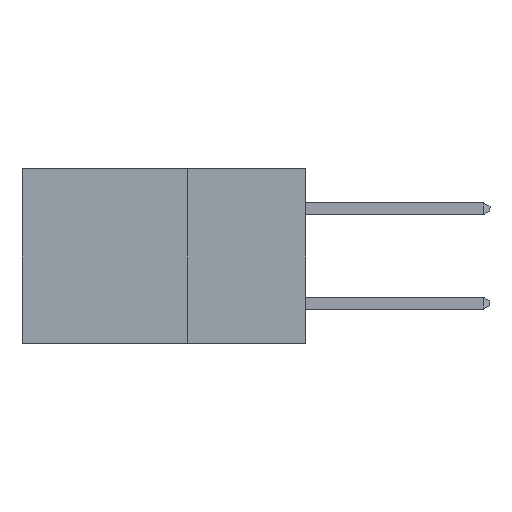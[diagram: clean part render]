
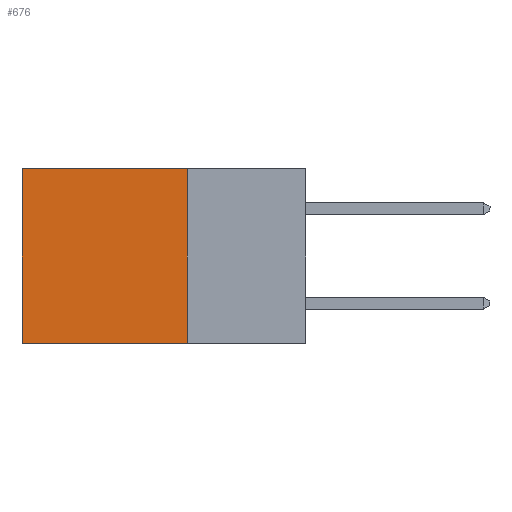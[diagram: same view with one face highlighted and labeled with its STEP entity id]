
A CAD part, left-side view. The second image highlights one B-rep face of the part: STEP entity #676.
In plain terms, the highlighted planar face has unit normal (-1, 0, 0).
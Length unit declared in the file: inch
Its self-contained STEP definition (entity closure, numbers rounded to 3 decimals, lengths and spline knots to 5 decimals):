
#16 = ORIENTED_EDGE ( 'NONE', *, *, #1226, .T. ) ;
#355 = CARTESIAN_POINT ( 'NONE',  ( 0.2615, 0.25, -0.37 ) ) ;
#676 = ADVANCED_FACE ( 'NONE', ( #8545 ), #761, .F. ) ;
#695 = VERTEX_POINT ( 'NONE', #2772 ) ;
#712 = LINE ( 'NONE', #3366, #1003 ) ;
#761 = PLANE ( 'NONE',  #7669 ) ;
#1003 = VECTOR ( 'NONE', #4851, 39.37008 ) ;
#1226 = EDGE_CURVE ( 'NONE', #3999, #4444, #6048, .T. ) ;
#1452 = EDGE_CURVE ( 'NONE', #3999, #8250, #7833, .T. ) ;
#2411 = EDGE_CURVE ( 'NONE', #4444, #695, #3205, .T. ) ;
#2772 = CARTESIAN_POINT ( 'NONE',  ( 0.2615, 0.6, -0.37 ) ) ;
#3035 = ORIENTED_EDGE ( 'NONE', *, *, #2411, .T. ) ;
#3205 = LINE ( 'NONE', #8413, #6080 ) ;
#3366 = CARTESIAN_POINT ( 'NONE',  ( 0.2615, 0.25, -0.37 ) ) ;
#3568 = DIRECTION ( 'NONE',  ( 0., 1., 0. ) ) ;
#3773 = CARTESIAN_POINT ( 'NONE',  ( 0.2615, 0.25, 0. ) ) ;
#3919 = CARTESIAN_POINT ( 'NONE',  ( 0.2615, 0.25, -0.37 ) ) ;
#3999 = VERTEX_POINT ( 'NONE', #3773 ) ;
#4074 = DIRECTION ( 'NONE',  ( 1., 0., 0. ) ) ;
#4093 = CARTESIAN_POINT ( 'NONE',  ( 0.2615, 0.25, 0. ) ) ;
#4444 = VERTEX_POINT ( 'NONE', #4496 ) ;
#4496 = CARTESIAN_POINT ( 'NONE',  ( 0.2615, 0.6, 0. ) ) ;
#4619 = DIRECTION ( 'NONE',  ( 0., 0., -1. ) ) ;
#4690 = DIRECTION ( 'NONE',  ( 0., 0., -1. ) ) ;
#4851 = DIRECTION ( 'NONE',  ( 0., 1., 0. ) ) ;
#5490 = VECTOR ( 'NONE', #3568, 39.37008 ) ;
#5857 = DIRECTION ( 'NONE',  ( 0., 0., -1. ) ) ;
#6013 = VECTOR ( 'NONE', #4619, 39.37008 ) ;
#6048 = LINE ( 'NONE', #4093, #5490 ) ;
#6080 = VECTOR ( 'NONE', #5857, 39.37008 ) ;
#6112 = CARTESIAN_POINT ( 'NONE',  ( 0.2615, 0.25, -0.37 ) ) ;
#6800 = EDGE_CURVE ( 'NONE', #8250, #695, #712, .T. ) ;
#6832 = EDGE_LOOP ( 'NONE', ( #3035, #8511, #8141, #16 ) ) ;
#7669 = AXIS2_PLACEMENT_3D ( 'NONE', #6112, #4074, #4690 ) ;
#7833 = LINE ( 'NONE', #3919, #6013 ) ;
#8141 = ORIENTED_EDGE ( 'NONE', *, *, #1452, .F. ) ;
#8250 = VERTEX_POINT ( 'NONE', #355 ) ;
#8413 = CARTESIAN_POINT ( 'NONE',  ( 0.2615, 0.6, -0.37 ) ) ;
#8511 = ORIENTED_EDGE ( 'NONE', *, *, #6800, .F. ) ;
#8545 = FACE_OUTER_BOUND ( 'NONE', #6832, .T. ) ;
